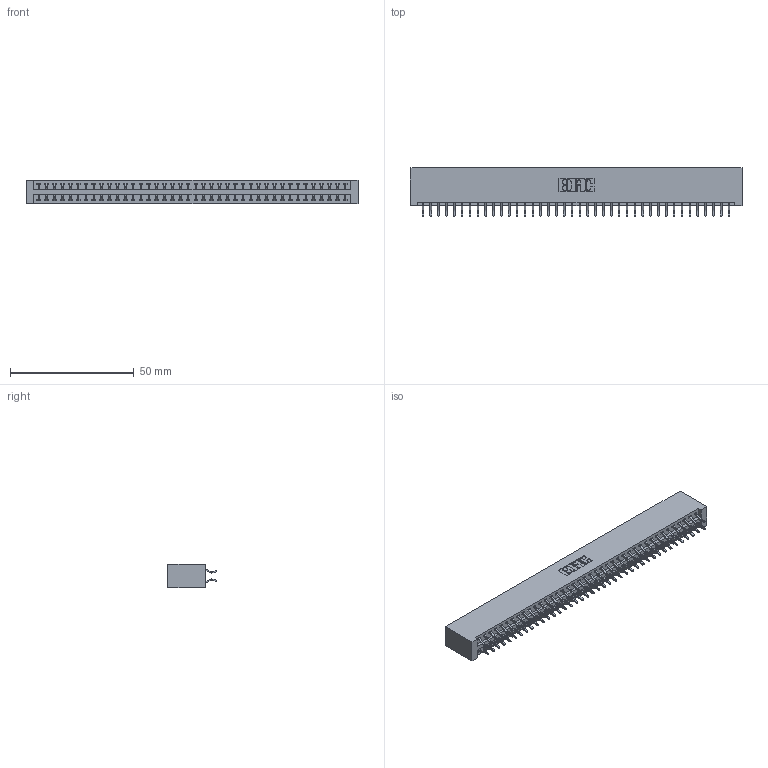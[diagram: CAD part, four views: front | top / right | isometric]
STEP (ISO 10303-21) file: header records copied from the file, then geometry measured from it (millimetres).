
FILE_DESCRIPTION (( 'STEP AP203' ), '1' );
FILE_NAME ('396-080-556-201.STEP', '2019-10-30T23:04:03', ( '' ), ( '' ), 'SwSTEP 2.0', 'SolidWorks 2016', '' );
FILE_SCHEMA (( 'CONFIG_CONTROL_DESIGN' ));
Length unit declared in the file: inch
Products named in the file (3): 396-080-556-201; 346 Part_No Mounting Lugs; 345-292-001_556 Tail
Assembly tree (81 placements, depth 2):
  396-080-556-201
    346 Part_No Mounting Lugs
    345-292-001_556 Tail  x80
Bounding box: 134.24 x 19.57 x 9.4 mm (x, y, z)
Volume: 13644.6 mm3; surface area: 18812.8 mm2
Topology: 81 solids, 81 shells, 4754 faces, 14145 edges, 9322 vertices
Faces by surface type: plane 3192, cylinder 1562
Entity records: 26317 total; most frequent: CARTESIAN_POINT 4352, ORIENTED_EDGE 4274, DIRECTION 3869, EDGE_CURVE 2137, LINE 1845, VECTOR 1845, VERTEX_POINT 1422, AXIS2_PLACEMENT_3D 1012
